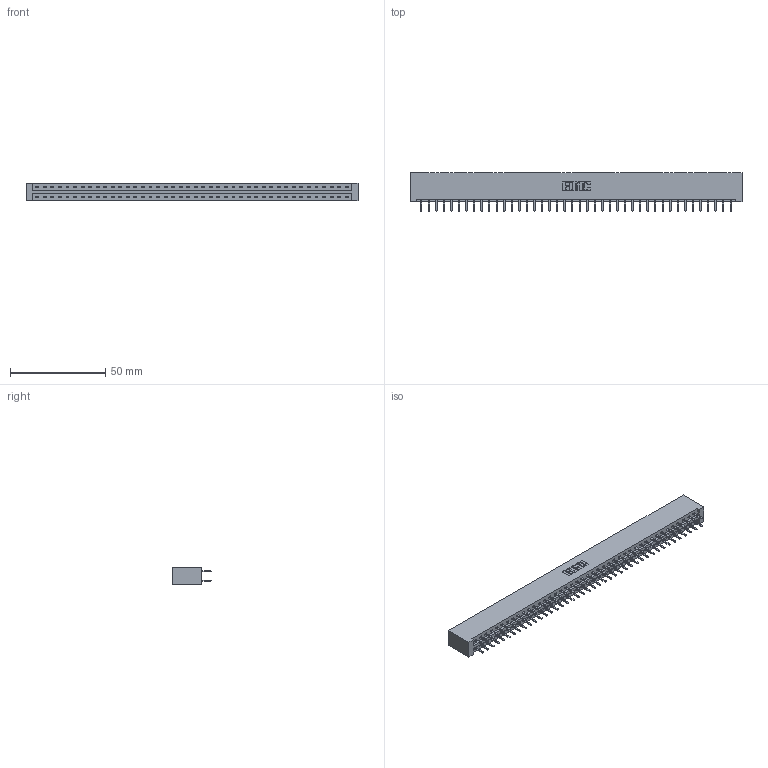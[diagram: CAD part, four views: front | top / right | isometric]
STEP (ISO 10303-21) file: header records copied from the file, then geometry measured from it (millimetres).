
FILE_DESCRIPTION (( 'STEP AP203' ), '1' );
FILE_NAME ('387-084-520-201.STEP', '2018-09-23T21:17:50', ( '' ), ( '' ), 'SwSTEP 2.0', 'SolidWorks 2016', '' );
FILE_SCHEMA (( 'CONFIG_CONTROL_DESIGN' ));
Length unit declared in the file: inch
Products named in the file (3): 337 Part_No Mounting Lugs; 345-292-001_345-293-120; 387-084-520-201
Assembly tree (85 placements, depth 2):
  387-084-520-201
    337 Part_No Mounting Lugs
    345-292-001_345-293-120  x84
Bounding box: 174.29 x 20.02 x 9.4 mm (x, y, z)
Volume: 19092.4 mm3; surface area: 21534.7 mm2
Topology: 85 solids, 85 shells, 4978 faces, 14483 edges, 9430 vertices
Faces by surface type: plane 3426, cylinder 1552
Entity records: 32401 total; most frequent: CARTESIAN_POINT 5470, ORIENTED_EDGE 5394, DIRECTION 4633, EDGE_CURVE 2697, VECTOR 2573, LINE 2573, VERTEX_POINT 1794, AXIS2_PLACEMENT_3D 1030
